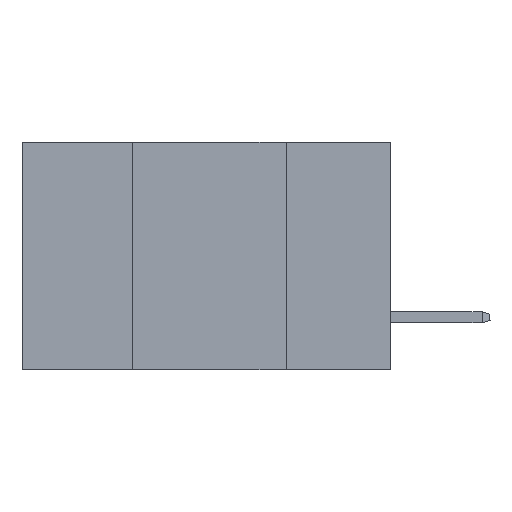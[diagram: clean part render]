
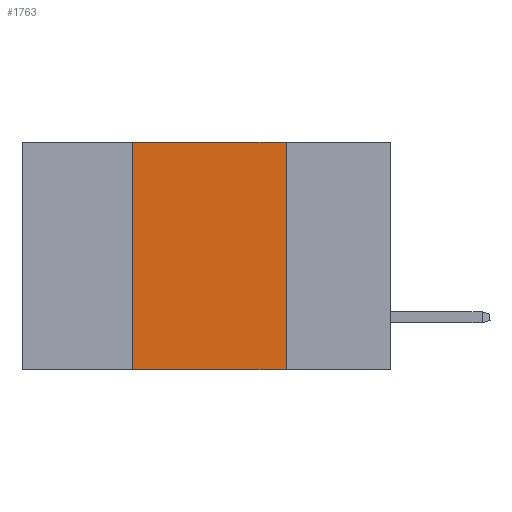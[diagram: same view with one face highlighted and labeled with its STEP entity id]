
A CAD part, left-side view. The second image highlights one B-rep face of the part: STEP entity #1763.
In plain terms, the highlighted planar face has unit normal (-1, 0, 0).
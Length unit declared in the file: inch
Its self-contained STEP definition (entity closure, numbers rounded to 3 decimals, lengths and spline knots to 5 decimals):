
#260 = AXIS2_PLACEMENT_3D ( 'NONE', #22103, #6763, #18942 ) ;
#807 = PLANE ( 'NONE',  #260 ) ;
#1763 = ADVANCED_FACE ( 'NONE', ( #15257 ), #807, .F. ) ;
#3187 = CARTESIAN_POINT ( 'NONE',  ( 0., 0.17, 0. ) ) ;
#4941 = LINE ( 'NONE', #3187, #10626 ) ;
#6763 = DIRECTION ( 'NONE',  ( 1., 0., 0. ) ) ;
#6951 = LINE ( 'NONE', #15394, #28730 ) ;
#9449 = CARTESIAN_POINT ( 'NONE',  ( 0., 0.17, -0.37 ) ) ;
#10626 = VECTOR ( 'NONE', #30427, 39.37008 ) ;
#10851 = VERTEX_POINT ( 'NONE', #14821 ) ;
#11227 = DIRECTION ( 'NONE',  ( 0., 0., 1. ) ) ;
#12624 = CARTESIAN_POINT ( 'NONE',  ( 0., 0.42, 0. ) ) ;
#14821 = CARTESIAN_POINT ( 'NONE',  ( 0., 0.17, 0. ) ) ;
#15257 = FACE_OUTER_BOUND ( 'NONE', #37421, .T. ) ;
#15394 = CARTESIAN_POINT ( 'NONE',  ( 0., 0.6, -0.37 ) ) ;
#18942 = DIRECTION ( 'NONE',  ( 0., 0., -1. ) ) ;
#19245 = CARTESIAN_POINT ( 'NONE',  ( 0., 0.42, -0.37 ) ) ;
#21852 = DIRECTION ( 'NONE',  ( 0., -1., 0. ) ) ;
#22103 = CARTESIAN_POINT ( 'NONE',  ( 0., 0.6, 0. ) ) ;
#22267 = EDGE_CURVE ( 'NONE', #26387, #10851, #37666, .T. ) ;
#22310 = ORIENTED_EDGE ( 'NONE', *, *, #34716, .F. ) ;
#23075 = ORIENTED_EDGE ( 'NONE', *, *, #28142, .T. ) ;
#24417 = VERTEX_POINT ( 'NONE', #19245 ) ;
#24452 = VECTOR ( 'NONE', #21852, 39.37008 ) ;
#26387 = VERTEX_POINT ( 'NONE', #12624 ) ;
#28142 = EDGE_CURVE ( 'NONE', #24417, #35597, #6951, .T. ) ;
#28730 = VECTOR ( 'NONE', #30734, 39.37008 ) ;
#29826 = ORIENTED_EDGE ( 'NONE', *, *, #29877, .F. ) ;
#29877 = EDGE_CURVE ( 'NONE', #10851, #35597, #4941, .T. ) ;
#30427 = DIRECTION ( 'NONE',  ( 0., 0., -1. ) ) ;
#30734 = DIRECTION ( 'NONE',  ( 0., -1., 0. ) ) ;
#32984 = VECTOR ( 'NONE', #11227, 39.37008 ) ;
#33109 = CARTESIAN_POINT ( 'NONE',  ( 0., 0.6, 0. ) ) ;
#34716 = EDGE_CURVE ( 'NONE', #24417, #26387, #34893, .T. ) ;
#34893 = LINE ( 'NONE', #38329, #32984 ) ;
#35597 = VERTEX_POINT ( 'NONE', #9449 ) ;
#37421 = EDGE_LOOP ( 'NONE', ( #29826, #37557, #22310, #23075 ) ) ;
#37557 = ORIENTED_EDGE ( 'NONE', *, *, #22267, .F. ) ;
#37666 = LINE ( 'NONE', #33109, #24452 ) ;
#38329 = CARTESIAN_POINT ( 'NONE',  ( 0., 0.42, 0. ) ) ;
